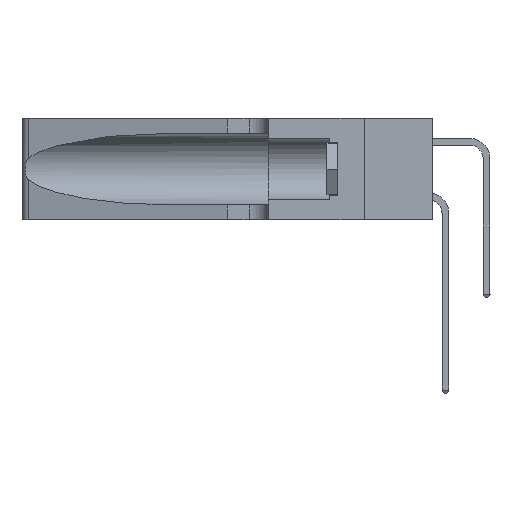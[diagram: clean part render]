
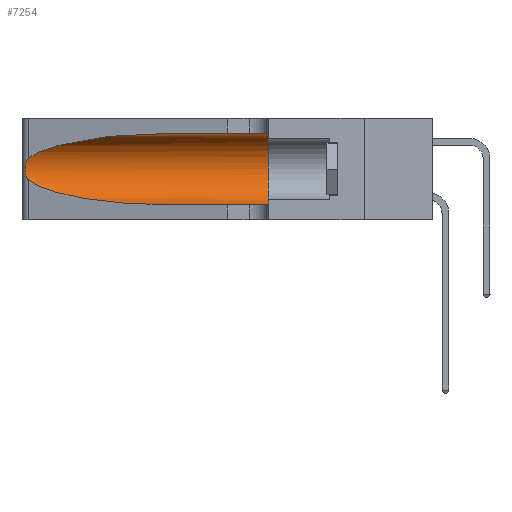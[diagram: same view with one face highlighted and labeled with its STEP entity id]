
A CAD part, left-side view. The second image highlights one B-rep face of the part: STEP entity #7254.
In plain terms, the highlighted cylindrical face has radius 3.308 mm (diameter 6.617 mm), a partial arc.
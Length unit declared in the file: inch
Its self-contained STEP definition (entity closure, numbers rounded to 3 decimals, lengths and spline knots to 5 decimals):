
#184 = CARTESIAN_POINT ( 'NONE',  ( 0.25854, 1.2359, 0.20912 ) ) ;
#239 = CARTESIAN_POINT ( 'NONE',  ( 0.1305, 0.35, 0.185 ) ) ;
#962 = CARTESIAN_POINT ( 'NONE',  ( 0.1305, 0.72297, 0.31525 ) ) ;
#1522 = VERTEX_POINT ( 'NONE', #12258 ) ;
#1884 = B_SPLINE_CURVE_WITH_KNOTS ( 'NONE', 3,
 ( #8895, #19285, #21008, #10714, #184, #12464, #1976, #14177, #3762, #15891, #5525, #17634, #7267, #19360 ),
 .UNSPECIFIED., .F., .F.,
 ( 4, 2, 2, 2, 2, 2, 4 ),
 ( 0., 0.00027, 0.00053, 0.00107, 0.0016, 0.00187, 0.00214 ),
 .UNSPECIFIED. ) ;
#1976 = CARTESIAN_POINT ( 'NONE',  ( 0.26075, 1.23896, 0.19203 ) ) ;
#2023 = DIRECTION ( 'NONE',  ( 0., 0., 1. ) ) ;
#2336 = CARTESIAN_POINT ( 'NONE',  ( 0.18966, 0.96281, 0.31525 ) ) ;
#2578 =( BOUNDED_CURVE ( )  B_SPLINE_CURVE ( 3, ( #18030, #19741, #9438, #21481 ),
 .UNSPECIFIED., .F., .T. ) 
 B_SPLINE_CURVE_WITH_KNOTS ( ( 4, 4 ),
 ( 3.44316, 4.71239 ),
 .UNSPECIFIED. ) 
 CURVE ( )  GEOMETRIC_REPRESENTATION_ITEM ( )  RATIONAL_B_SPLINE_CURVE ( ( 1., 0.87, 0.87, 1. ) ) 
 REPRESENTATION_ITEM ( '' )  );
#2788 = CARTESIAN_POINT ( 'NONE',  ( 0.25487, 1.22718, 0.14631 ) ) ;
#3141 = CARTESIAN_POINT ( 'NONE',  ( 0.1305, 1.61858, 0.31525 ) ) ;
#3597 = CYLINDRICAL_SURFACE ( 'NONE', #18555, 0.13025 ) ;
#3762 = CARTESIAN_POINT ( 'NONE',  ( 0.26017, 1.23833, 0.17102 ) ) ;
#3910 = ORIENTED_EDGE ( 'NONE', *, *, #11988, .T. ) ;
#4997 =( BOUNDED_CURVE ( )  B_SPLINE_CURVE ( 3, ( #14541, #2336, #17989, #7622 ),
 .UNSPECIFIED., .F., .F. ) 
 B_SPLINE_CURVE_WITH_KNOTS ( ( 4, 4 ),
 ( 1.5708, 2.84003 ),
 .UNSPECIFIED. ) 
 CURVE ( )  GEOMETRIC_REPRESENTATION_ITEM ( )  RATIONAL_B_SPLINE_CURVE ( ( 1., 0.87, 0.87, 1. ) ) 
 REPRESENTATION_ITEM ( '' )  );
#5309 = VECTOR ( 'NONE', #15121, 39.37008 ) ;
#5525 = CARTESIAN_POINT ( 'NONE',  ( 0.25789, 1.23486, 0.15765 ) ) ;
#5871 = EDGE_CURVE ( 'NONE', #10487, #1522, #10733, .T. ) ;
#6083 = VERTEX_POINT ( 'NONE', #8951 ) ;
#6090 = VECTOR ( 'NONE', #22203, 39.37008 ) ;
#6280 = CIRCLE ( 'NONE', #9469, 0.13025 ) ;
#6397 = LINE ( 'NONE', #13421, #5309 ) ;
#7254 = ADVANCED_FACE ( 'NONE', ( #12866 ), #3597, .F. ) ;
#7267 = CARTESIAN_POINT ( 'NONE',  ( 0.25555, 1.22993, 0.14849 ) ) ;
#7372 = ORIENTED_EDGE ( 'NONE', *, *, #21287, .T. ) ;
#7622 = CARTESIAN_POINT ( 'NONE',  ( 0.25487, 1.22718, 0.22369 ) ) ;
#8795 = CARTESIAN_POINT ( 'NONE',  ( 0.1305, 0.35, 0.05475 ) ) ;
#8895 = CARTESIAN_POINT ( 'NONE',  ( 0.25487, 1.22718, 0.22369 ) ) ;
#8951 = CARTESIAN_POINT ( 'NONE',  ( 0.25487, 1.22718, 0.22369 ) ) ;
#9194 = VERTEX_POINT ( 'NONE', #2788 ) ;
#9438 = CARTESIAN_POINT ( 'NONE',  ( 0.18966, 0.96281, 0.05475 ) ) ;
#9469 = AXIS2_PLACEMENT_3D ( 'NONE', #239, #12512, #2023 ) ;
#10487 = VERTEX_POINT ( 'NONE', #962 ) ;
#10584 = DIRECTION ( 'NONE',  ( 0., 0., -1. ) ) ;
#10714 = CARTESIAN_POINT ( 'NONE',  ( 0.25787, 1.23484, 0.2124 ) ) ;
#10733 = LINE ( 'NONE', #3141, #6090 ) ;
#11748 = EDGE_CURVE ( 'NONE', #10487, #6083, #4997, .T. ) ;
#11801 = ORIENTED_EDGE ( 'NONE', *, *, #5871, .F. ) ;
#11988 = EDGE_CURVE ( 'NONE', #19226, #19294, #6397, .T. ) ;
#12258 = CARTESIAN_POINT ( 'NONE',  ( 0.1305, 0.35, 0.31525 ) ) ;
#12464 = CARTESIAN_POINT ( 'NONE',  ( 0.26018, 1.23835, 0.19895 ) ) ;
#12512 = DIRECTION ( 'NONE',  ( 0., 1., 0. ) ) ;
#12866 = FACE_OUTER_BOUND ( 'NONE', #13631, .T. ) ;
#13421 = CARTESIAN_POINT ( 'NONE',  ( 0.1305, 1.61858, 0.05475 ) ) ;
#13631 = EDGE_LOOP ( 'NONE', ( #19520, #15413, #7372, #3910, #22079, #11801 ) ) ;
#14177 = CARTESIAN_POINT ( 'NONE',  ( 0.26075, 1.23896, 0.178 ) ) ;
#14541 = CARTESIAN_POINT ( 'NONE',  ( 0.1305, 0.72297, 0.31525 ) ) ;
#15121 = DIRECTION ( 'NONE',  ( 0., -1., 0. ) ) ;
#15413 = ORIENTED_EDGE ( 'NONE', *, *, #21763, .T. ) ;
#15891 = CARTESIAN_POINT ( 'NONE',  ( 0.25856, 1.23593, 0.16098 ) ) ;
#17184 = CARTESIAN_POINT ( 'NONE',  ( 0.1305, 0.72297, 0.05475 ) ) ;
#17634 = CARTESIAN_POINT ( 'NONE',  ( 0.25639, 1.23186, 0.15144 ) ) ;
#17989 = CARTESIAN_POINT ( 'NONE',  ( 0.2373, 1.15595, 0.28018 ) ) ;
#18030 = CARTESIAN_POINT ( 'NONE',  ( 0.25487, 1.22718, 0.14631 ) ) ;
#18555 = AXIS2_PLACEMENT_3D ( 'NONE', #19159, #20879, #10584 ) ;
#19159 = CARTESIAN_POINT ( 'NONE',  ( 0.1305, 1.61858, 0.185 ) ) ;
#19226 = VERTEX_POINT ( 'NONE', #17184 ) ;
#19285 = CARTESIAN_POINT ( 'NONE',  ( 0.25555, 1.22994, 0.2215 ) ) ;
#19294 = VERTEX_POINT ( 'NONE', #8795 ) ;
#19360 = CARTESIAN_POINT ( 'NONE',  ( 0.25487, 1.22718, 0.14631 ) ) ;
#19376 = EDGE_CURVE ( 'NONE', #1522, #19294, #6280, .T. ) ;
#19520 = ORIENTED_EDGE ( 'NONE', *, *, #11748, .T. ) ;
#19741 = CARTESIAN_POINT ( 'NONE',  ( 0.2373, 1.15595, 0.08982 ) ) ;
#20879 = DIRECTION ( 'NONE',  ( 0., -1., 0. ) ) ;
#21008 = CARTESIAN_POINT ( 'NONE',  ( 0.25639, 1.23184, 0.21858 ) ) ;
#21287 = EDGE_CURVE ( 'NONE', #9194, #19226, #2578, .T. ) ;
#21481 = CARTESIAN_POINT ( 'NONE',  ( 0.1305, 0.72297, 0.05475 ) ) ;
#21763 = EDGE_CURVE ( 'NONE', #6083, #9194, #1884, .T. ) ;
#22079 = ORIENTED_EDGE ( 'NONE', *, *, #19376, .F. ) ;
#22203 = DIRECTION ( 'NONE',  ( 0., -1., 0. ) ) ;
